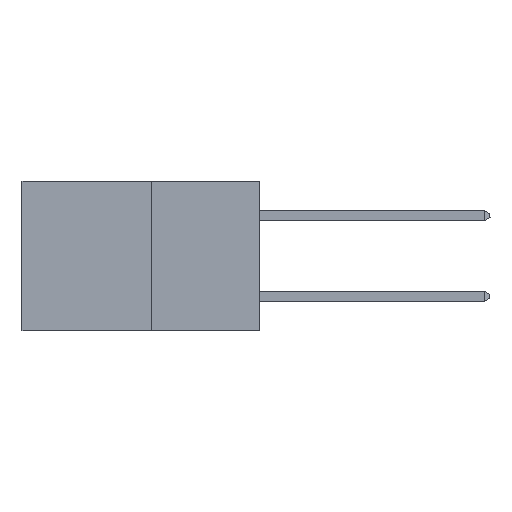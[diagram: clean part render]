
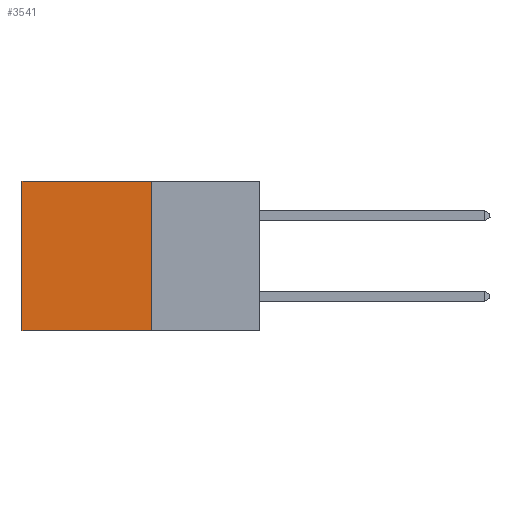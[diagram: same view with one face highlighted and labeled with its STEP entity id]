
A CAD part, left-side view. The second image highlights one B-rep face of the part: STEP entity #3541.
In plain terms, the highlighted planar face has unit normal (-1, 0, 0).
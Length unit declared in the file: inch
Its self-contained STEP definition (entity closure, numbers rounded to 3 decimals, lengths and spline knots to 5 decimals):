
#1072 = VERTEX_POINT ( 'NONE', #5807 ) ;
#1225 = DIRECTION ( 'NONE',  ( 0., 0., -1. ) ) ;
#2156 = DIRECTION ( 'NONE',  ( 0., 1., 0. ) ) ;
#2679 = CARTESIAN_POINT ( 'NONE',  ( 0.277, 0.27, -0.37 ) ) ;
#2887 = LINE ( 'NONE', #32010, #14963 ) ;
#3411 = ORIENTED_EDGE ( 'NONE', *, *, #26725, .F. ) ;
#3541 = ADVANCED_FACE ( 'NONE', ( #21943 ), #15513, .F. ) ;
#3556 = VERTEX_POINT ( 'NONE', #25854 ) ;
#4409 = VERTEX_POINT ( 'NONE', #31718 ) ;
#4774 = CARTESIAN_POINT ( 'NONE',  ( 0.277, 0.27, -0.37 ) ) ;
#5250 = EDGE_CURVE ( 'NONE', #4409, #3556, #2887, .T. ) ;
#5292 = DIRECTION ( 'NONE',  ( 0., 0., -1. ) ) ;
#5807 = CARTESIAN_POINT ( 'NONE',  ( 0.277, 0.59, 0. ) ) ;
#7217 = VERTEX_POINT ( 'NONE', #7235 ) ;
#7235 = CARTESIAN_POINT ( 'NONE',  ( 0.277, 0.59, -0.37 ) ) ;
#9843 = ORIENTED_EDGE ( 'NONE', *, *, #5250, .F. ) ;
#11344 = VECTOR ( 'NONE', #2156, 39.37008 ) ;
#14120 = ORIENTED_EDGE ( 'NONE', *, *, #18356, .T. ) ;
#14267 = VECTOR ( 'NONE', #27062, 39.37008 ) ;
#14278 = CARTESIAN_POINT ( 'NONE',  ( 0.277, 0.59, -0.37 ) ) ;
#14963 = VECTOR ( 'NONE', #1225, 39.37008 ) ;
#15513 = PLANE ( 'NONE',  #29508 ) ;
#17505 = VECTOR ( 'NONE', #27039, 39.37008 ) ;
#17785 = EDGE_CURVE ( 'NONE', #4409, #1072, #18321, .T. ) ;
#18321 = LINE ( 'NONE', #19302, #17505 ) ;
#18356 = EDGE_CURVE ( 'NONE', #1072, #7217, #21875, .T. ) ;
#19302 = CARTESIAN_POINT ( 'NONE',  ( 0.277, 0.27, 0. ) ) ;
#20667 = DIRECTION ( 'NONE',  ( 1., 0., 0. ) ) ;
#21875 = LINE ( 'NONE', #14278, #14267 ) ;
#21943 = FACE_OUTER_BOUND ( 'NONE', #31124, .T. ) ;
#25299 = LINE ( 'NONE', #4774, #11344 ) ;
#25854 = CARTESIAN_POINT ( 'NONE',  ( 0.277, 0.27, -0.37 ) ) ;
#26725 = EDGE_CURVE ( 'NONE', #3556, #7217, #25299, .T. ) ;
#27039 = DIRECTION ( 'NONE',  ( 0., 1., 0. ) ) ;
#27062 = DIRECTION ( 'NONE',  ( 0., 0., -1. ) ) ;
#29508 = AXIS2_PLACEMENT_3D ( 'NONE', #2679, #20667, #5292 ) ;
#30707 = ORIENTED_EDGE ( 'NONE', *, *, #17785, .T. ) ;
#31124 = EDGE_LOOP ( 'NONE', ( #14120, #3411, #9843, #30707 ) ) ;
#31718 = CARTESIAN_POINT ( 'NONE',  ( 0.277, 0.27, 0. ) ) ;
#32010 = CARTESIAN_POINT ( 'NONE',  ( 0.277, 0.27, -0.37 ) ) ;
